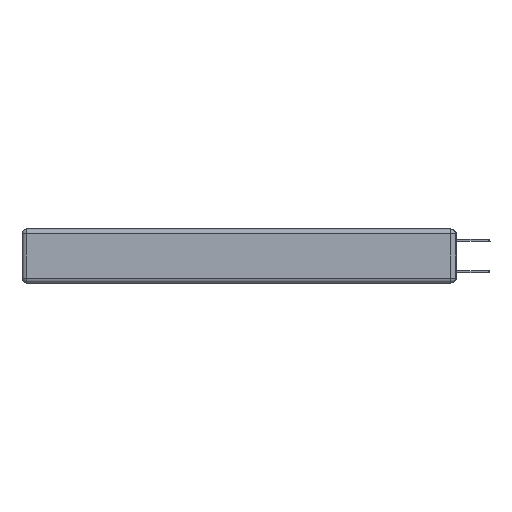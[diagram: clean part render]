
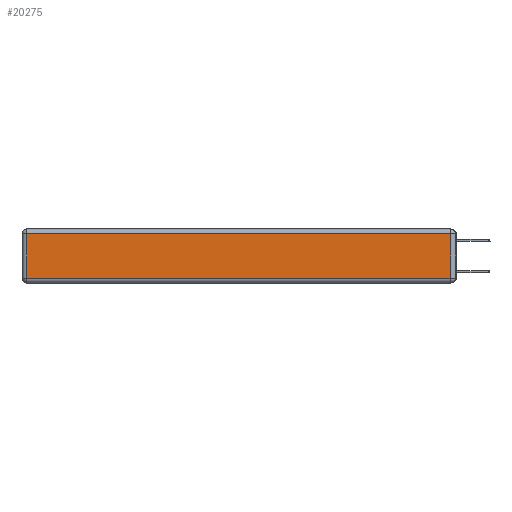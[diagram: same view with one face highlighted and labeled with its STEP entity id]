
A CAD part, left-side view. The second image highlights one B-rep face of the part: STEP entity #20275.
In plain terms, the highlighted planar face has unit normal (-1, 0, 0).
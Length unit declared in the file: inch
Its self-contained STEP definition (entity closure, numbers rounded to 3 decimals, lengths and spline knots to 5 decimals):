
#43 = CARTESIAN_POINT ( 'NONE',  ( 0., 0.03, -0.343 ) ) ;
#593 = CARTESIAN_POINT ( 'NONE',  ( 0., 2.72, -0.03 ) ) ;
#1033 = ORIENTED_EDGE ( 'NONE', *, *, #12117, .T. ) ;
#2054 = CARTESIAN_POINT ( 'NONE',  ( 0., 0.03, -0.03 ) ) ;
#2185 = CARTESIAN_POINT ( 'NONE',  ( 0., 0., -0.313 ) ) ;
#2201 = CARTESIAN_POINT ( 'NONE',  ( 0., 2.75, -0.03 ) ) ;
#2586 = CARTESIAN_POINT ( 'NONE',  ( 0., 0.03, -0.313 ) ) ;
#2930 = LINE ( 'NONE', #14450, #6550 ) ;
#4460 = ORIENTED_EDGE ( 'NONE', *, *, #6615, .T. ) ;
#4799 = PLANE ( 'NONE',  #11605 ) ;
#5356 = DIRECTION ( 'NONE',  ( 0., -1., 0. ) ) ;
#5516 = EDGE_CURVE ( 'NONE', #10913, #16085, #10349, .T. ) ;
#6173 = DIRECTION ( 'NONE',  ( -1., 0., 0. ) ) ;
#6351 = EDGE_CURVE ( 'NONE', #6633, #9383, #15079, .T. ) ;
#6550 = VECTOR ( 'NONE', #7689, 39.37008 ) ;
#6615 = EDGE_CURVE ( 'NONE', #9383, #10913, #9781, .T. ) ;
#6633 = VERTEX_POINT ( 'NONE', #16143 ) ;
#6765 = ORIENTED_EDGE ( 'NONE', *, *, #5516, .T. ) ;
#7527 = VECTOR ( 'NONE', #16345, 39.37008 ) ;
#7689 = DIRECTION ( 'NONE',  ( 0., 0., -1. ) ) ;
#9176 = VECTOR ( 'NONE', #16802, 39.37008 ) ;
#9383 = VERTEX_POINT ( 'NONE', #2586 ) ;
#9781 = LINE ( 'NONE', #43, #7527 ) ;
#10349 = LINE ( 'NONE', #2201, #9176 ) ;
#10913 = VERTEX_POINT ( 'NONE', #2054 ) ;
#11605 = AXIS2_PLACEMENT_3D ( 'NONE', #20703, #6173, #18894 ) ;
#12117 = EDGE_CURVE ( 'NONE', #16085, #6633, #2930, .T. ) ;
#14450 = CARTESIAN_POINT ( 'NONE',  ( 0., 2.72, -0.343 ) ) ;
#15079 = LINE ( 'NONE', #2185, #20054 ) ;
#15819 = FACE_OUTER_BOUND ( 'NONE', #19341, .T. ) ;
#16085 = VERTEX_POINT ( 'NONE', #593 ) ;
#16143 = CARTESIAN_POINT ( 'NONE',  ( 0., 2.72, -0.313 ) ) ;
#16345 = DIRECTION ( 'NONE',  ( 0., 0., 1. ) ) ;
#16802 = DIRECTION ( 'NONE',  ( 0., 1., 0. ) ) ;
#18894 = DIRECTION ( 'NONE',  ( 0., 0., 1. ) ) ;
#19341 = EDGE_LOOP ( 'NONE', ( #19575, #4460, #6765, #1033 ) ) ;
#19575 = ORIENTED_EDGE ( 'NONE', *, *, #6351, .T. ) ;
#20054 = VECTOR ( 'NONE', #5356, 39.37008 ) ;
#20275 = ADVANCED_FACE ( 'NONE', ( #15819 ), #4799, .T. ) ;
#20703 = CARTESIAN_POINT ( 'NONE',  ( 0., 0., -0.343 ) ) ;
